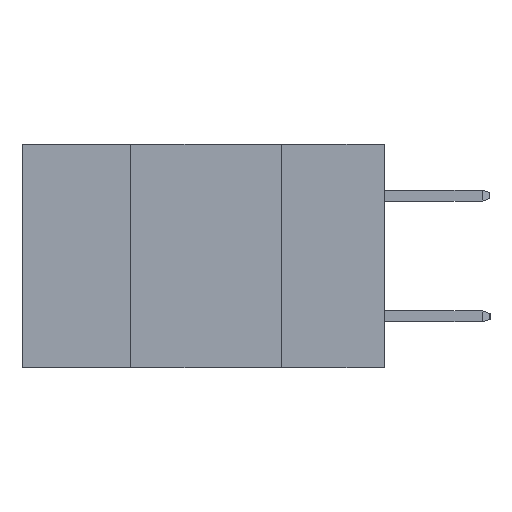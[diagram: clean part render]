
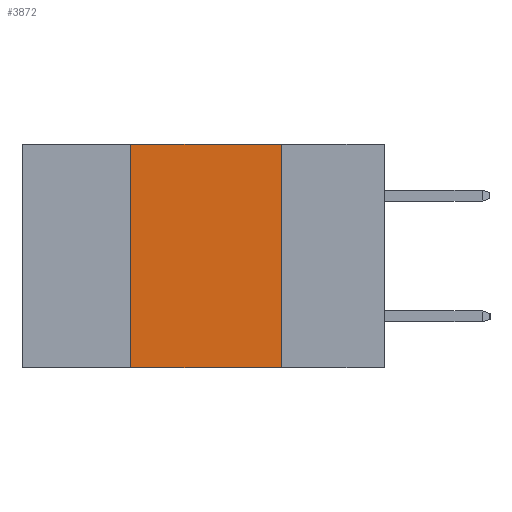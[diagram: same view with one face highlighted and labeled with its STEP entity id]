
A CAD part, left-side view. The second image highlights one B-rep face of the part: STEP entity #3872.
In plain terms, the highlighted planar face has unit normal (-1, 0, 0).
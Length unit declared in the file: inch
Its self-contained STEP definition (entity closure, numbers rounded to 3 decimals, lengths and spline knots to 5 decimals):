
#1479 = CARTESIAN_POINT ( 'NONE',  ( 0., 0.6, -0.37 ) ) ;
#1694 = AXIS2_PLACEMENT_3D ( 'NONE', #2124, #2046, #1977 ) ;
#1977 = DIRECTION ( 'NONE',  ( 0., 0., -1. ) ) ;
#2046 = DIRECTION ( 'NONE',  ( 1., 0., 0. ) ) ;
#2102 = VERTEX_POINT ( 'NONE', #10008 ) ;
#2124 = CARTESIAN_POINT ( 'NONE',  ( 0., 0.6, 0. ) ) ;
#2383 = PLANE ( 'NONE',  #1694 ) ;
#2899 = CARTESIAN_POINT ( 'NONE',  ( 0., 0.6, 0. ) ) ;
#3006 = VERTEX_POINT ( 'NONE', #7522 ) ;
#3687 = EDGE_CURVE ( 'NONE', #6724, #2102, #8605, .T. ) ;
#3819 = CARTESIAN_POINT ( 'NONE',  ( 0., 0.17, 0. ) ) ;
#3872 = ADVANCED_FACE ( 'NONE', ( #5765 ), #2383, .F. ) ;
#4488 = CARTESIAN_POINT ( 'NONE',  ( 0., 0.42, -0.37 ) ) ;
#5426 = EDGE_LOOP ( 'NONE', ( #5698, #5747, #5826, #5838 ) ) ;
#5697 = DIRECTION ( 'NONE',  ( 0., 0., 1. ) ) ;
#5698 = ORIENTED_EDGE ( 'NONE', *, *, #3687, .F. ) ;
#5747 = ORIENTED_EDGE ( 'NONE', *, *, #6848, .F. ) ;
#5765 = FACE_OUTER_BOUND ( 'NONE', #5426, .T. ) ;
#5826 = ORIENTED_EDGE ( 'NONE', *, *, #9835, .F. ) ;
#5838 = ORIENTED_EDGE ( 'NONE', *, *, #7308, .T. ) ;
#6724 = VERTEX_POINT ( 'NONE', #3819 ) ;
#6848 = EDGE_CURVE ( 'NONE', #12568, #6724, #8349, .T. ) ;
#6965 = LINE ( 'NONE', #1479, #9924 ) ;
#7308 = EDGE_CURVE ( 'NONE', #3006, #2102, #6965, .T. ) ;
#7522 = CARTESIAN_POINT ( 'NONE',  ( 0., 0.42, -0.37 ) ) ;
#8349 = LINE ( 'NONE', #2899, #14233 ) ;
#8605 = LINE ( 'NONE', #11239, #11267 ) ;
#9835 = EDGE_CURVE ( 'NONE', #3006, #12568, #14325, .T. ) ;
#9924 = VECTOR ( 'NONE', #10565, 39.37008 ) ;
#10008 = CARTESIAN_POINT ( 'NONE',  ( 0., 0.17, -0.37 ) ) ;
#10565 = DIRECTION ( 'NONE',  ( 0., -1., 0. ) ) ;
#10767 = DIRECTION ( 'NONE',  ( 0., 0., -1. ) ) ;
#10881 = DIRECTION ( 'NONE',  ( 0., -1., 0. ) ) ;
#11096 = VECTOR ( 'NONE', #5697, 39.37008 ) ;
#11239 = CARTESIAN_POINT ( 'NONE',  ( 0., 0.17, -0.37 ) ) ;
#11267 = VECTOR ( 'NONE', #10767, 39.37008 ) ;
#12568 = VERTEX_POINT ( 'NONE', #13629 ) ;
#13629 = CARTESIAN_POINT ( 'NONE',  ( 0., 0.42, 0. ) ) ;
#14233 = VECTOR ( 'NONE', #10881, 39.37008 ) ;
#14325 = LINE ( 'NONE', #4488, #11096 ) ;
